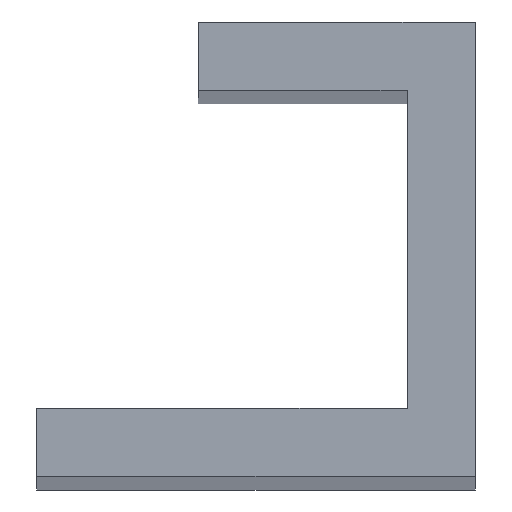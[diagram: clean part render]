
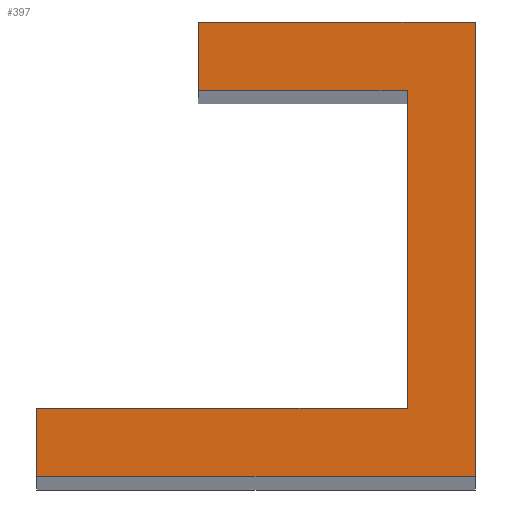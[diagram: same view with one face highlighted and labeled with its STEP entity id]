
A CAD part, top view. The second image highlights one B-rep face of the part: STEP entity #397.
In plain terms, the highlighted planar face has unit normal (0, 0, 1).
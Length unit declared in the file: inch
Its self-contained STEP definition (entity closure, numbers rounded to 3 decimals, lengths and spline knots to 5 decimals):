
#63=FACE_OUTER_BOUND('',#81,.T.);
#81=EDGE_LOOP('',(#275,#276,#277,#278,#279,#280,#281,#282));
#115=LINE('',#599,#147);
#116=LINE('',#601,#148);
#117=LINE('',#603,#149);
#118=LINE('',#605,#150);
#119=LINE('',#607,#151);
#120=LINE('',#609,#152);
#121=LINE('',#611,#153);
#122=LINE('',#612,#154);
#147=VECTOR('',#481,0.3937);
#148=VECTOR('',#482,0.3937);
#149=VECTOR('',#483,0.3937);
#150=VECTOR('',#484,0.3937);
#151=VECTOR('',#485,0.3937);
#152=VECTOR('',#486,0.3937);
#153=VECTOR('',#487,0.3937);
#154=VECTOR('',#488,0.3937);
#179=VERTEX_POINT('',#597);
#180=VERTEX_POINT('',#598);
#181=VERTEX_POINT('',#600);
#182=VERTEX_POINT('',#602);
#183=VERTEX_POINT('',#604);
#184=VERTEX_POINT('',#606);
#185=VERTEX_POINT('',#608);
#186=VERTEX_POINT('',#610);
#219=EDGE_CURVE('',#179,#180,#115,.T.);
#220=EDGE_CURVE('',#181,#179,#116,.T.);
#221=EDGE_CURVE('',#182,#181,#117,.T.);
#222=EDGE_CURVE('',#183,#182,#118,.T.);
#223=EDGE_CURVE('',#184,#183,#119,.T.);
#224=EDGE_CURVE('',#185,#184,#120,.T.);
#225=EDGE_CURVE('',#186,#185,#121,.T.);
#226=EDGE_CURVE('',#180,#186,#122,.T.);
#275=ORIENTED_EDGE('',*,*,#219,.F.);
#276=ORIENTED_EDGE('',*,*,#220,.F.);
#277=ORIENTED_EDGE('',*,*,#221,.F.);
#278=ORIENTED_EDGE('',*,*,#222,.F.);
#279=ORIENTED_EDGE('',*,*,#223,.F.);
#280=ORIENTED_EDGE('',*,*,#224,.F.);
#281=ORIENTED_EDGE('',*,*,#225,.F.);
#282=ORIENTED_EDGE('',*,*,#226,.F.);
#387=PLANE('',#435);
#397=ADVANCED_FACE('',(#63),#387,.F.);
#435=AXIS2_PLACEMENT_3D('',#596,#479,#480);
#479=DIRECTION('center_axis',(0.,0.,-1.));
#480=DIRECTION('ref_axis',(-1.,0.,0.));
#481=DIRECTION('',(0.,1.,0.));
#482=DIRECTION('',(-1.,0.,0.));
#483=DIRECTION('',(0.,1.,0.));
#484=DIRECTION('',(1.,0.,0.));
#485=DIRECTION('',(0.,1.,0.));
#486=DIRECTION('',(-1.,0.,0.));
#487=DIRECTION('',(0.,-1.,0.));
#488=DIRECTION('',(1.,0.,0.));
#596=CARTESIAN_POINT('Origin',(0.19,0.19685,6.80194));
#597=CARTESIAN_POINT('',(0.14,0.33465,6.80194));
#598=CARTESIAN_POINT('',(0.14,0.3937,6.80194));
#599=CARTESIAN_POINT('',(0.14,0.26575,6.80194));
#600=CARTESIAN_POINT('',(0.32094,0.33465,6.80194));
#601=CARTESIAN_POINT('',(0.145,0.33465,6.80194));
#602=CARTESIAN_POINT('',(0.32094,0.05906,6.80194));
#603=CARTESIAN_POINT('',(0.32094,0.26575,6.80194));
#604=CARTESIAN_POINT('',(0.,0.05906,6.80194));
#605=CARTESIAN_POINT('',(0.25547,0.05906,6.80194));
#606=CARTESIAN_POINT('',(0.,0.,6.80194));
#607=CARTESIAN_POINT('',(0.,0.12795,6.80194));
#608=CARTESIAN_POINT('',(0.38,0.,6.80194));
#609=CARTESIAN_POINT('',(0.095,0.,6.80194));
#610=CARTESIAN_POINT('',(0.38,0.3937,6.80194));
#611=CARTESIAN_POINT('',(0.38,0.09843,6.80194));
#612=CARTESIAN_POINT('',(0.285,0.3937,6.80194));
